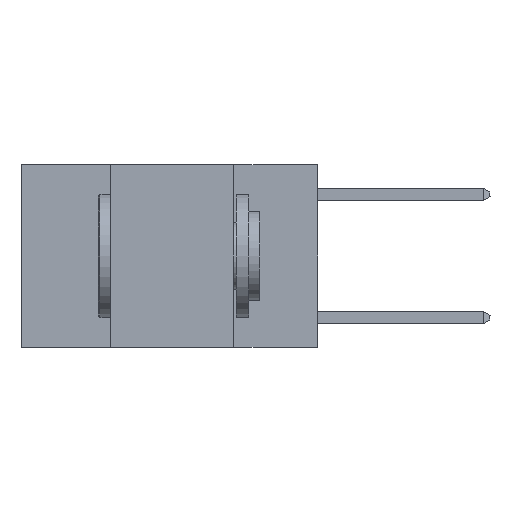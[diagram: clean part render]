
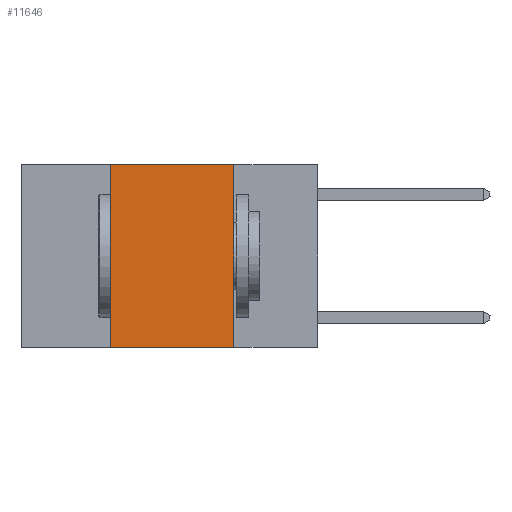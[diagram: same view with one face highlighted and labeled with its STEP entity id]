
A CAD part, left-side view. The second image highlights one B-rep face of the part: STEP entity #11646.
In plain terms, the highlighted planar face has unit normal (-1, 0, 0).
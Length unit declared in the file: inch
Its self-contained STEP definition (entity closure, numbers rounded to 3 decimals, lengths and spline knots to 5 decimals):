
#993 = CARTESIAN_POINT ( 'NONE',  ( 0., 0.17, 0. ) ) ;
#2248 = VERTEX_POINT ( 'NONE', #8267 ) ;
#3756 = EDGE_CURVE ( 'NONE', #15347, #28312, #4467, .T. ) ;
#4467 = LINE ( 'NONE', #11188, #7062 ) ;
#4770 = LINE ( 'NONE', #15932, #7976 ) ;
#4799 = DIRECTION ( 'NONE',  ( 0., -1., 0. ) ) ;
#5655 = ORIENTED_EDGE ( 'NONE', *, *, #20861, .F. ) ;
#7062 = VECTOR ( 'NONE', #27872, 39.37008 ) ;
#7602 = ORIENTED_EDGE ( 'NONE', *, *, #3756, .F. ) ;
#7976 = VECTOR ( 'NONE', #18224, 39.37008 ) ;
#8267 = CARTESIAN_POINT ( 'NONE',  ( 0., 0.42, -0.37 ) ) ;
#9818 = DIRECTION ( 'NONE',  ( 1., 0., 0. ) ) ;
#11188 = CARTESIAN_POINT ( 'NONE',  ( 0., 0.17, 0. ) ) ;
#11646 = ADVANCED_FACE ( 'NONE', ( #19013 ), #17155, .F. ) ;
#11977 = LINE ( 'NONE', #25743, #20753 ) ;
#15347 = VERTEX_POINT ( 'NONE', #993 ) ;
#15932 = CARTESIAN_POINT ( 'NONE',  ( 0., 0.6, -0.37 ) ) ;
#16096 = EDGE_CURVE ( 'NONE', #2248, #28312, #4770, .T. ) ;
#16121 = CARTESIAN_POINT ( 'NONE',  ( 0., 0.42, 0. ) ) ;
#17155 = PLANE ( 'NONE',  #28750 ) ;
#17789 = ORIENTED_EDGE ( 'NONE', *, *, #16096, .T. ) ;
#18224 = DIRECTION ( 'NONE',  ( 0., -1., 0. ) ) ;
#19013 = FACE_OUTER_BOUND ( 'NONE', #25586, .T. ) ;
#20688 = VERTEX_POINT ( 'NONE', #16121 ) ;
#20753 = VECTOR ( 'NONE', #4799, 39.37008 ) ;
#20861 = EDGE_CURVE ( 'NONE', #20688, #15347, #11977, .T. ) ;
#22793 = CARTESIAN_POINT ( 'NONE',  ( 0., 0.42, 0. ) ) ;
#24076 = ORIENTED_EDGE ( 'NONE', *, *, #29854, .F. ) ;
#24625 = LINE ( 'NONE', #22793, #27830 ) ;
#25586 = EDGE_LOOP ( 'NONE', ( #7602, #5655, #24076, #17789 ) ) ;
#25721 = CARTESIAN_POINT ( 'NONE',  ( 0., 0.17, -0.37 ) ) ;
#25743 = CARTESIAN_POINT ( 'NONE',  ( 0., 0.6, 0. ) ) ;
#26497 = CARTESIAN_POINT ( 'NONE',  ( 0., 0.6, 0. ) ) ;
#27537 = DIRECTION ( 'NONE',  ( 0., 0., 1. ) ) ;
#27830 = VECTOR ( 'NONE', #27537, 39.37008 ) ;
#27872 = DIRECTION ( 'NONE',  ( 0., 0., -1. ) ) ;
#28312 = VERTEX_POINT ( 'NONE', #25721 ) ;
#28367 = DIRECTION ( 'NONE',  ( 0., 0., -1. ) ) ;
#28750 = AXIS2_PLACEMENT_3D ( 'NONE', #26497, #9818, #28367 ) ;
#29854 = EDGE_CURVE ( 'NONE', #2248, #20688, #24625, .T. ) ;
